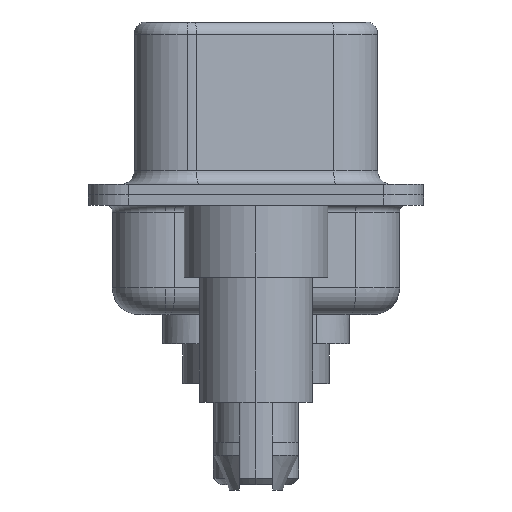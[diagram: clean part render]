
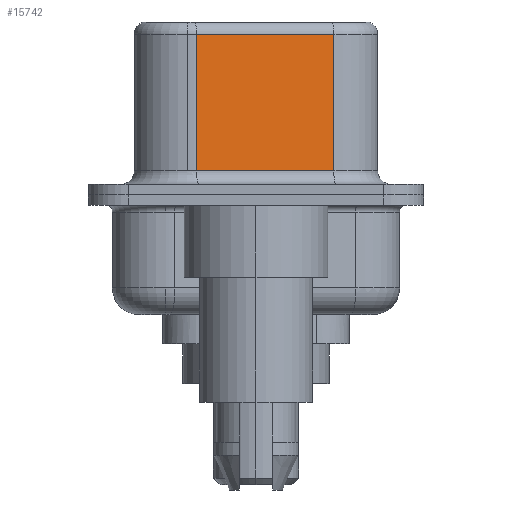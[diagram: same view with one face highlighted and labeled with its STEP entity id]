
A CAD part, left-side view. The second image highlights one B-rep face of the part: STEP entity #15742.
In plain terms, the highlighted planar face has unit normal (-0.985, -0.174, 0).
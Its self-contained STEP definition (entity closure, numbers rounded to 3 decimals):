
#380 = DIRECTION ( 'NONE',  ( 0.174, -0.985, 0. ) ) ;
#1848 = CARTESIAN_POINT ( 'NONE',  ( 4.58, -2.927, 6.02 ) ) ;
#1940 = VERTEX_POINT ( 'NONE', #1848 ) ;
#2112 = LINE ( 'NONE', #13682, #17441 ) ;
#2227 = AXIS2_PLACEMENT_3D ( 'NONE', #13934, #12572, #3702 ) ;
#3544 = ORIENTED_EDGE ( 'NONE', *, *, #10513, .T. ) ;
#3683 = ORIENTED_EDGE ( 'NONE', *, *, #6675, .F. ) ;
#3702 = DIRECTION ( 'NONE',  ( -0.174, 0.985, 0. ) ) ;
#3979 = LINE ( 'NONE', #8827, #7094 ) ;
#4151 = ORIENTED_EDGE ( 'NONE', *, *, #9969, .T. ) ;
#4329 = FACE_OUTER_BOUND ( 'NONE', #6011, .T. ) ;
#5473 = CARTESIAN_POINT ( 'NONE',  ( 3.67, 2.233, 0.9 ) ) ;
#6011 = EDGE_LOOP ( 'NONE', ( #3683, #4151, #7815, #3544 ) ) ;
#6675 = EDGE_CURVE ( 'NONE', #1940, #11845, #3979, .T. ) ;
#7094 = VECTOR ( 'NONE', #9936, 1000. ) ;
#7400 = VERTEX_POINT ( 'NONE', #5473 ) ;
#7815 = ORIENTED_EDGE ( 'NONE', *, *, #12224, .T. ) ;
#7822 = DIRECTION ( 'NONE',  ( 0., 0., -1. ) ) ;
#8827 = CARTESIAN_POINT ( 'NONE',  ( 4.58, -2.927, 6.52 ) ) ;
#9936 = DIRECTION ( 'NONE',  ( 0., 0., -1. ) ) ;
#9943 = VECTOR ( 'NONE', #7822, 1000. ) ;
#9969 = EDGE_CURVE ( 'NONE', #1940, #16996, #16990, .T. ) ;
#10513 = EDGE_CURVE ( 'NONE', #7400, #11845, #2112, .T. ) ;
#11051 = PLANE ( 'NONE',  #2227 ) ;
#11845 = VERTEX_POINT ( 'NONE', #18942 ) ;
#12224 = EDGE_CURVE ( 'NONE', #16996, #7400, #17917, .T. ) ;
#12572 = DIRECTION ( 'NONE',  ( 0.985, 0.174, 0. ) ) ;
#13007 = VECTOR ( 'NONE', #18308, 1000. ) ;
#13682 = CARTESIAN_POINT ( 'NONE',  ( 4.58, -2.927, 0.9 ) ) ;
#13687 = CARTESIAN_POINT ( 'NONE',  ( 3.67, 2.233, 6.52 ) ) ;
#13934 = CARTESIAN_POINT ( 'NONE',  ( 4.58, -2.927, 6.52 ) ) ;
#15742 = ADVANCED_FACE ( 'NONE', ( #4329 ), #11051, .F. ) ;
#16620 = CARTESIAN_POINT ( 'NONE',  ( 3.67, 2.233, 6.02 ) ) ;
#16780 = CARTESIAN_POINT ( 'NONE',  ( 4.58, -2.927, 6.02 ) ) ;
#16990 = LINE ( 'NONE', #16780, #13007 ) ;
#16996 = VERTEX_POINT ( 'NONE', #16620 ) ;
#17441 = VECTOR ( 'NONE', #380, 1000. ) ;
#17917 = LINE ( 'NONE', #13687, #9943 ) ;
#18308 = DIRECTION ( 'NONE',  ( -0.174, 0.985, 0. ) ) ;
#18942 = CARTESIAN_POINT ( 'NONE',  ( 4.58, -2.927, 0.9 ) ) ;
